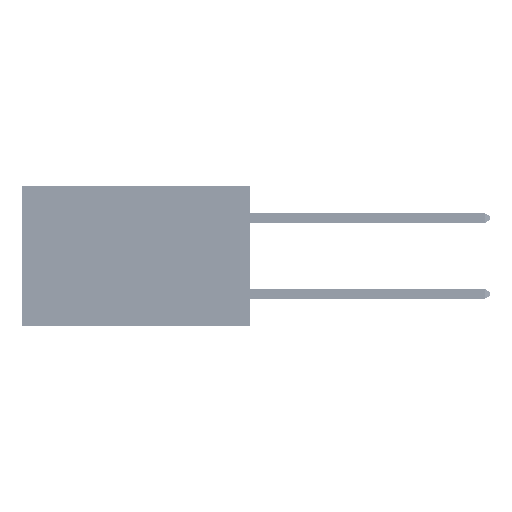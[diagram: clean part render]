
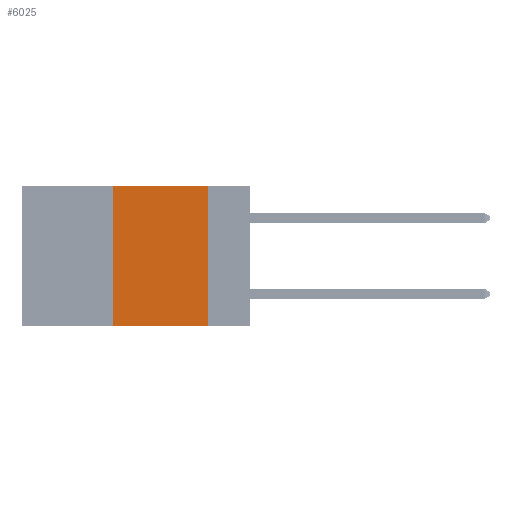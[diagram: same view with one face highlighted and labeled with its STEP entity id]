
A CAD part, left-side view. The second image highlights one B-rep face of the part: STEP entity #6025.
In plain terms, the highlighted planar face has unit normal (-1, 0, 0).
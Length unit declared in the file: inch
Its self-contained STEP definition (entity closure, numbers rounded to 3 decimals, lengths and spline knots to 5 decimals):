
#37 = CARTESIAN_POINT ( 'NONE',  ( 0., 0.11, 0. ) ) ;
#1280 = EDGE_CURVE ( 'NONE', #45126, #31733, #43761, .T. ) ;
#6025 = ADVANCED_FACE ( 'NONE', ( #50515 ), #39128, .F. ) ;
#6103 = VECTOR ( 'NONE', #44161, 39.37008 ) ;
#7329 = DIRECTION ( 'NONE',  ( 0., 0., -1. ) ) ;
#7727 = AXIS2_PLACEMENT_3D ( 'NONE', #39637, #34995, #7329 ) ;
#8331 = EDGE_CURVE ( 'NONE', #48434, #45126, #28640, .T. ) ;
#9312 = CARTESIAN_POINT ( 'NONE',  ( 0., 0.36, 0. ) ) ;
#11131 = CARTESIAN_POINT ( 'NONE',  ( 0., 0.6, -0.37 ) ) ;
#18319 = CARTESIAN_POINT ( 'NONE',  ( 0., 0.11, -0.37 ) ) ;
#18553 = VECTOR ( 'NONE', #19962, 39.37008 ) ;
#19157 = CARTESIAN_POINT ( 'NONE',  ( 0., 0.36, 0. ) ) ;
#19897 = CARTESIAN_POINT ( 'NONE',  ( 0., 0.36, -0.37 ) ) ;
#19962 = DIRECTION ( 'NONE',  ( 0., 0., -1. ) ) ;
#23011 = DIRECTION ( 'NONE',  ( 0., -1., 0. ) ) ;
#24395 = EDGE_CURVE ( 'NONE', #29643, #48434, #50963, .T. ) ;
#25480 = CARTESIAN_POINT ( 'NONE',  ( 0., 0.11, 0. ) ) ;
#27879 = CARTESIAN_POINT ( 'NONE',  ( 0., 0.6, 0. ) ) ;
#28640 = LINE ( 'NONE', #27879, #6103 ) ;
#29643 = VERTEX_POINT ( 'NONE', #19897 ) ;
#31391 = EDGE_CURVE ( 'NONE', #29643, #31733, #46563, .T. ) ;
#31733 = VERTEX_POINT ( 'NONE', #18319 ) ;
#34995 = DIRECTION ( 'NONE',  ( 1., 0., 0. ) ) ;
#37281 = ORIENTED_EDGE ( 'NONE', *, *, #1280, .F. ) ;
#38700 = ORIENTED_EDGE ( 'NONE', *, *, #31391, .T. ) ;
#39128 = PLANE ( 'NONE',  #7727 ) ;
#39637 = CARTESIAN_POINT ( 'NONE',  ( 0., 0.6, 0. ) ) ;
#43761 = LINE ( 'NONE', #37, #18553 ) ;
#44161 = DIRECTION ( 'NONE',  ( 0., -1., 0. ) ) ;
#44457 = ORIENTED_EDGE ( 'NONE', *, *, #8331, .F. ) ;
#44968 = ORIENTED_EDGE ( 'NONE', *, *, #24395, .F. ) ;
#45126 = VERTEX_POINT ( 'NONE', #25480 ) ;
#46563 = LINE ( 'NONE', #11131, #46904 ) ;
#46835 = DIRECTION ( 'NONE',  ( 0., 0., 1. ) ) ;
#46904 = VECTOR ( 'NONE', #23011, 39.37008 ) ;
#48434 = VERTEX_POINT ( 'NONE', #9312 ) ;
#50515 = FACE_OUTER_BOUND ( 'NONE', #50876, .T. ) ;
#50563 = VECTOR ( 'NONE', #46835, 39.37008 ) ;
#50876 = EDGE_LOOP ( 'NONE', ( #37281, #44457, #44968, #38700 ) ) ;
#50963 = LINE ( 'NONE', #19157, #50563 ) ;
